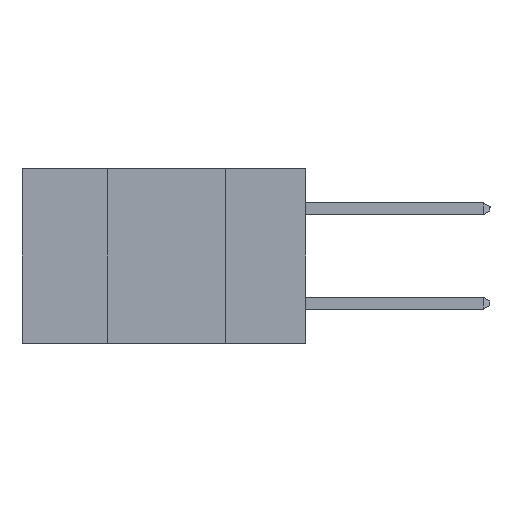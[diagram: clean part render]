
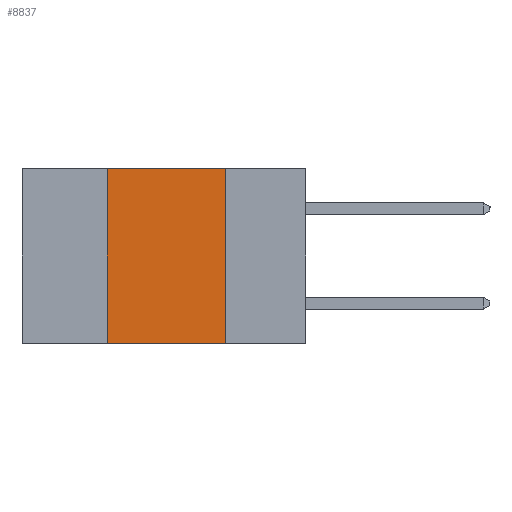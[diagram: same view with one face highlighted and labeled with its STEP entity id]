
A CAD part, left-side view. The second image highlights one B-rep face of the part: STEP entity #8837.
In plain terms, the highlighted planar face has unit normal (-1, 0, 0).
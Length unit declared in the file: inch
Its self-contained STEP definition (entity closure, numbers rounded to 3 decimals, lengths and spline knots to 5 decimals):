
#345 = ORIENTED_EDGE ( 'NONE', *, *, #1261, .F. ) ;
#813 = ORIENTED_EDGE ( 'NONE', *, *, #3132, .T. ) ;
#942 = CARTESIAN_POINT ( 'NONE',  ( 0., 0.6, -0.37 ) ) ;
#1261 = EDGE_CURVE ( 'NONE', #10596, #7067, #9493, .T. ) ;
#1484 = VECTOR ( 'NONE', #8517, 39.37008 ) ;
#1538 = CARTESIAN_POINT ( 'NONE',  ( 0., 0.42, 0. ) ) ;
#2771 = CARTESIAN_POINT ( 'NONE',  ( 0., 0.17, -0.37 ) ) ;
#3132 = EDGE_CURVE ( 'NONE', #8138, #7067, #9436, .T. ) ;
#3592 = ORIENTED_EDGE ( 'NONE', *, *, #7435, .F. ) ;
#3655 = LINE ( 'NONE', #11953, #10231 ) ;
#3819 = VERTEX_POINT ( 'NONE', #1538 ) ;
#4160 = PLANE ( 'NONE',  #4393 ) ;
#4393 = AXIS2_PLACEMENT_3D ( 'NONE', #10595, #11864, #10725 ) ;
#5604 = CARTESIAN_POINT ( 'NONE',  ( 0., 0.6, 0. ) ) ;
#5825 = ORIENTED_EDGE ( 'NONE', *, *, #10411, .F. ) ;
#6703 = DIRECTION ( 'NONE',  ( 0., 0., 1. ) ) ;
#7067 = VERTEX_POINT ( 'NONE', #12390 ) ;
#7435 = EDGE_CURVE ( 'NONE', #8138, #3819, #3655, .T. ) ;
#7873 = LINE ( 'NONE', #5604, #10040 ) ;
#8114 = VECTOR ( 'NONE', #12626, 39.37008 ) ;
#8138 = VERTEX_POINT ( 'NONE', #13903 ) ;
#8517 = DIRECTION ( 'NONE',  ( 0., -1., 0. ) ) ;
#8837 = ADVANCED_FACE ( 'NONE', ( #9177 ), #4160, .F. ) ;
#9177 = FACE_OUTER_BOUND ( 'NONE', #12357, .T. ) ;
#9436 = LINE ( 'NONE', #942, #1484 ) ;
#9493 = LINE ( 'NONE', #2771, #8114 ) ;
#10040 = VECTOR ( 'NONE', #12189, 39.37008 ) ;
#10231 = VECTOR ( 'NONE', #6703, 39.37008 ) ;
#10411 = EDGE_CURVE ( 'NONE', #3819, #10596, #7873, .T. ) ;
#10595 = CARTESIAN_POINT ( 'NONE',  ( 0., 0.6, 0. ) ) ;
#10596 = VERTEX_POINT ( 'NONE', #13870 ) ;
#10725 = DIRECTION ( 'NONE',  ( 0., 0., -1. ) ) ;
#11864 = DIRECTION ( 'NONE',  ( 1., 0., 0. ) ) ;
#11953 = CARTESIAN_POINT ( 'NONE',  ( 0., 0.42, -0.37 ) ) ;
#12189 = DIRECTION ( 'NONE',  ( 0., -1., 0. ) ) ;
#12357 = EDGE_LOOP ( 'NONE', ( #345, #5825, #3592, #813 ) ) ;
#12390 = CARTESIAN_POINT ( 'NONE',  ( 0., 0.17, -0.37 ) ) ;
#12626 = DIRECTION ( 'NONE',  ( 0., 0., -1. ) ) ;
#13870 = CARTESIAN_POINT ( 'NONE',  ( 0., 0.17, 0. ) ) ;
#13903 = CARTESIAN_POINT ( 'NONE',  ( 0., 0.42, -0.37 ) ) ;
